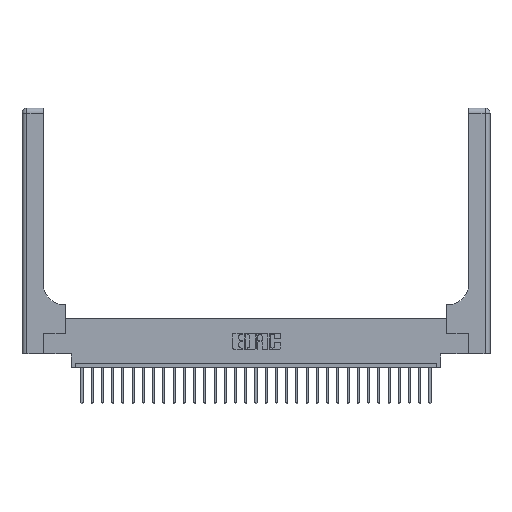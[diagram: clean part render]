
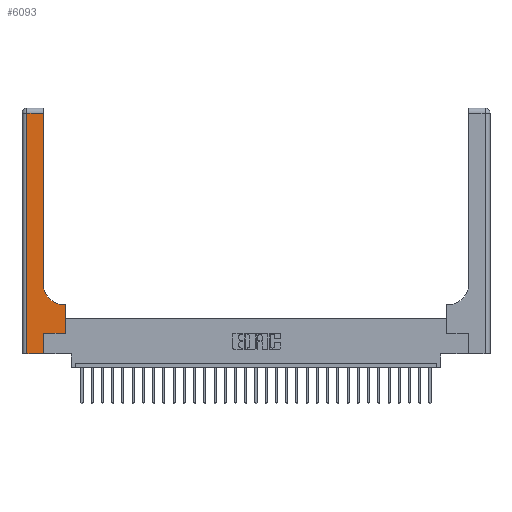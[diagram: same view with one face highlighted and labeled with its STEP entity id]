
A CAD part, top view. The second image highlights one B-rep face of the part: STEP entity #6093.
In plain terms, the highlighted planar face has unit normal (0, 0, 1).
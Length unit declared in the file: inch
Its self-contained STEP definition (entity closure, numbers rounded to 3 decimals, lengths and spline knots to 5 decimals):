
#1017 = ORIENTED_EDGE ( 'NONE', *, *, #16405, .T. ) ;
#1231 = CARTESIAN_POINT ( 'NONE',  ( 0.06, 2.94, 0.37 ) ) ;
#1442 = CARTESIAN_POINT ( 'NONE',  ( 0.51, 0.6, 0.37 ) ) ;
#1617 = VERTEX_POINT ( 'NONE', #11773 ) ;
#2173 = VECTOR ( 'NONE', #16317, 39.37008 ) ;
#3812 = DIRECTION ( 'NONE',  ( 0., 0., -1. ) ) ;
#4024 = EDGE_CURVE ( 'NONE', #8056, #1617, #6349, .T. ) ;
#4346 = ORIENTED_EDGE ( 'NONE', *, *, #6351, .T. ) ;
#5300 = CARTESIAN_POINT ( 'NONE',  ( 0.265, 0.25, 0.37 ) ) ;
#5497 = EDGE_CURVE ( 'NONE', #27524, #7119, #20315, .T. ) ;
#5920 = ORIENTED_EDGE ( 'NONE', *, *, #16505, .T. ) ;
#6093 = ADVANCED_FACE ( 'NONE', ( #7140 ), #9025, .F. ) ;
#6349 = LINE ( 'NONE', #27817, #15328 ) ;
#6351 = EDGE_CURVE ( 'NONE', #24969, #8019, #15704, .T. ) ;
#7119 = VERTEX_POINT ( 'NONE', #16488 ) ;
#7140 = FACE_OUTER_BOUND ( 'NONE', #20617, .T. ) ;
#7149 = LINE ( 'NONE', #22267, #18195 ) ;
#7482 = LINE ( 'NONE', #5300, #23901 ) ;
#7844 = EDGE_CURVE ( 'NONE', #8019, #22747, #26175, .T. ) ;
#7921 = ORIENTED_EDGE ( 'NONE', *, *, #7844, .T. ) ;
#8019 = VERTEX_POINT ( 'NONE', #1442 ) ;
#8056 = VERTEX_POINT ( 'NONE', #14663 ) ;
#8156 = VECTOR ( 'NONE', #10486, 39.37008 ) ;
#8407 = DIRECTION ( 'NONE',  ( 1., 0., 0. ) ) ;
#8590 = VECTOR ( 'NONE', #10901, 39.37008 ) ;
#9025 = PLANE ( 'NONE',  #18992 ) ;
#9180 = VERTEX_POINT ( 'NONE', #15236 ) ;
#9384 = CARTESIAN_POINT ( 'NONE',  ( 0.06, 3., 0.37 ) ) ;
#10486 = DIRECTION ( 'NONE',  ( -1., 0., 0. ) ) ;
#10901 = DIRECTION ( 'NONE',  ( 1., 0., 0. ) ) ;
#11072 = LINE ( 'NONE', #16959, #8156 ) ;
#11683 = ORIENTED_EDGE ( 'NONE', *, *, #5497, .T. ) ;
#11773 = CARTESIAN_POINT ( 'NONE',  ( 0.265, 0.25, 0.37 ) ) ;
#12019 = LINE ( 'NONE', #16035, #2173 ) ;
#12100 = ORIENTED_EDGE ( 'NONE', *, *, #4024, .T. ) ;
#12780 = VECTOR ( 'NONE', #20015, 39.37008 ) ;
#13003 = ORIENTED_EDGE ( 'NONE', *, *, #19519, .T. ) ;
#13057 = CARTESIAN_POINT ( 'NONE',  ( 0.26, 2.94, 0.37 ) ) ;
#13944 = DIRECTION ( 'NONE',  ( 1., 0., 0. ) ) ;
#14095 = ORIENTED_EDGE ( 'NONE', *, *, #19992, .T. ) ;
#14584 = CARTESIAN_POINT ( 'NONE',  ( 0.528, 0.6, 0.37 ) ) ;
#14663 = CARTESIAN_POINT ( 'NONE',  ( 0.265, 0., 0.37 ) ) ;
#15102 = EDGE_CURVE ( 'NONE', #1617, #9180, #7482, .T. ) ;
#15218 = LINE ( 'NONE', #24013, #8590 ) ;
#15236 = CARTESIAN_POINT ( 'NONE',  ( 0.528, 0.25, 0.37 ) ) ;
#15328 = VECTOR ( 'NONE', #24061, 39.37008 ) ;
#15558 = CARTESIAN_POINT ( 'NONE',  ( 0.26, 0.6, 0.37 ) ) ;
#15704 = LINE ( 'NONE', #15558, #12780 ) ;
#16035 = CARTESIAN_POINT ( 'NONE',  ( 0.528, 0.25, 0.37 ) ) ;
#16317 = DIRECTION ( 'NONE',  ( 0., 1., 0. ) ) ;
#16405 = EDGE_CURVE ( 'NONE', #19475, #27524, #11072, .T. ) ;
#16488 = CARTESIAN_POINT ( 'NONE',  ( 0.06, 0., 0.37 ) ) ;
#16505 = EDGE_CURVE ( 'NONE', #22747, #19475, #7149, .T. ) ;
#16959 = CARTESIAN_POINT ( 'NONE',  ( 0., 2.94, 0.37 ) ) ;
#17279 = ORIENTED_EDGE ( 'NONE', *, *, #15102, .T. ) ;
#17550 = VECTOR ( 'NONE', #20013, 39.37008 ) ;
#17785 = DIRECTION ( 'NONE',  ( 0., 0., -1. ) ) ;
#18195 = VECTOR ( 'NONE', #22560, 39.37008 ) ;
#18992 = AXIS2_PLACEMENT_3D ( 'NONE', #26873, #17785, #24002 ) ;
#19046 = CARTESIAN_POINT ( 'NONE',  ( 0.51, 0.85, 0.37 ) ) ;
#19475 = VERTEX_POINT ( 'NONE', #13057 ) ;
#19519 = EDGE_CURVE ( 'NONE', #7119, #8056, #15218, .T. ) ;
#19992 = EDGE_CURVE ( 'NONE', #9180, #24969, #12019, .T. ) ;
#20013 = DIRECTION ( 'NONE',  ( 0., -1., 0. ) ) ;
#20015 = DIRECTION ( 'NONE',  ( -1., 0., 0. ) ) ;
#20315 = LINE ( 'NONE', #9384, #17550 ) ;
#20617 = EDGE_LOOP ( 'NONE', ( #5920, #1017, #11683, #13003, #12100, #17279, #14095, #4346, #7921 ) ) ;
#22267 = CARTESIAN_POINT ( 'NONE',  ( 0.26, 3., 0.37 ) ) ;
#22560 = DIRECTION ( 'NONE',  ( 0., 1., 0. ) ) ;
#22747 = VERTEX_POINT ( 'NONE', #23714 ) ;
#23714 = CARTESIAN_POINT ( 'NONE',  ( 0.26, 0.85, 0.37 ) ) ;
#23875 = AXIS2_PLACEMENT_3D ( 'NONE', #19046, #3812, #8407 ) ;
#23901 = VECTOR ( 'NONE', #13944, 39.37008 ) ;
#24002 = DIRECTION ( 'NONE',  ( -1., 0., 0. ) ) ;
#24013 = CARTESIAN_POINT ( 'NONE',  ( 0., 0., 0.37 ) ) ;
#24061 = DIRECTION ( 'NONE',  ( 0., 1., 0. ) ) ;
#24969 = VERTEX_POINT ( 'NONE', #14584 ) ;
#26175 = CIRCLE ( 'NONE', #23875, 0.25 ) ;
#26873 = CARTESIAN_POINT ( 'NONE',  ( 0., 3., 0.37 ) ) ;
#27524 = VERTEX_POINT ( 'NONE', #1231 ) ;
#27817 = CARTESIAN_POINT ( 'NONE',  ( 0.265, 0., 0.37 ) ) ;
